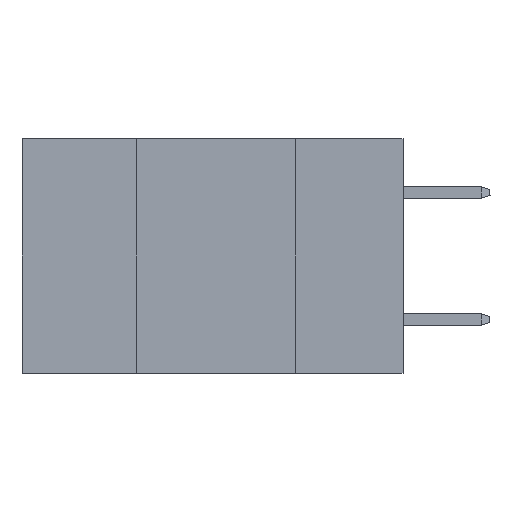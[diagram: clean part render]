
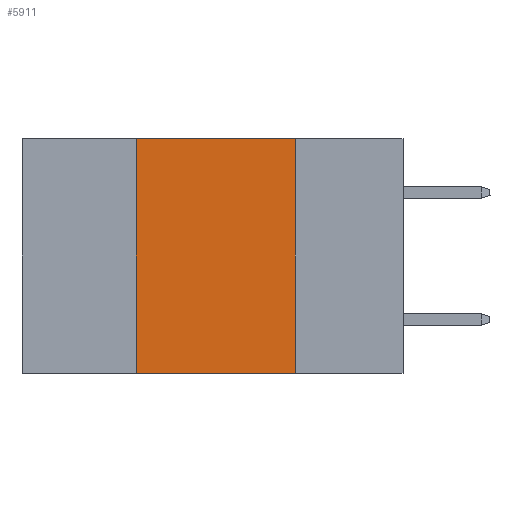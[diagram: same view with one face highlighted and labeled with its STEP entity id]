
A CAD part, left-side view. The second image highlights one B-rep face of the part: STEP entity #5911.
In plain terms, the highlighted planar face has unit normal (-1, 0, 0).
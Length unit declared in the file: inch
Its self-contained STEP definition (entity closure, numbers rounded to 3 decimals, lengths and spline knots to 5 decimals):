
#369 = CARTESIAN_POINT ( 'NONE',  ( 0., 0.42, -0.37 ) ) ;
#667 = VERTEX_POINT ( 'NONE', #26846 ) ;
#1873 = DIRECTION ( 'NONE',  ( 0., 0., 1. ) ) ;
#2934 = FACE_OUTER_BOUND ( 'NONE', #6196, .T. ) ;
#4989 = LINE ( 'NONE', #30145, #19191 ) ;
#5911 = ADVANCED_FACE ( 'NONE', ( #2934 ), #17420, .F. ) ;
#6111 = DIRECTION ( 'NONE',  ( 0., -1., 0. ) ) ;
#6196 = EDGE_LOOP ( 'NONE', ( #30304, #21961, #32910, #29564 ) ) ;
#7143 = EDGE_CURVE ( 'NONE', #31161, #16699, #19513, .T. ) ;
#8806 = DIRECTION ( 'NONE',  ( 1., 0., 0. ) ) ;
#11231 = CARTESIAN_POINT ( 'NONE',  ( 0., 0.17, -0.37 ) ) ;
#12310 = VECTOR ( 'NONE', #1873, 39.37008 ) ;
#16320 = CARTESIAN_POINT ( 'NONE',  ( 0., 0.6, -0.37 ) ) ;
#16699 = VERTEX_POINT ( 'NONE', #11231 ) ;
#17420 = PLANE ( 'NONE',  #36991 ) ;
#18185 = LINE ( 'NONE', #38845, #12310 ) ;
#19191 = VECTOR ( 'NONE', #22674, 39.37008 ) ;
#19513 = LINE ( 'NONE', #16320, #34757 ) ;
#21961 = ORIENTED_EDGE ( 'NONE', *, *, #22437, .F. ) ;
#22437 = EDGE_CURVE ( 'NONE', #667, #36093, #40378, .T. ) ;
#22674 = DIRECTION ( 'NONE',  ( 0., 0., -1. ) ) ;
#24629 = EDGE_CURVE ( 'NONE', #31161, #667, #18185, .T. ) ;
#24665 = CARTESIAN_POINT ( 'NONE',  ( 0., 0.17, 0. ) ) ;
#26737 = CARTESIAN_POINT ( 'NONE',  ( 0., 0.6, 0. ) ) ;
#26846 = CARTESIAN_POINT ( 'NONE',  ( 0., 0.42, 0. ) ) ;
#27868 = DIRECTION ( 'NONE',  ( 0., 0., -1. ) ) ;
#29564 = ORIENTED_EDGE ( 'NONE', *, *, #7143, .T. ) ;
#29944 = DIRECTION ( 'NONE',  ( 0., -1., 0. ) ) ;
#30145 = CARTESIAN_POINT ( 'NONE',  ( 0., 0.17, 0. ) ) ;
#30304 = ORIENTED_EDGE ( 'NONE', *, *, #35763, .F. ) ;
#31161 = VERTEX_POINT ( 'NONE', #369 ) ;
#32910 = ORIENTED_EDGE ( 'NONE', *, *, #24629, .F. ) ;
#34757 = VECTOR ( 'NONE', #29944, 39.37008 ) ;
#35763 = EDGE_CURVE ( 'NONE', #36093, #16699, #4989, .T. ) ;
#36093 = VERTEX_POINT ( 'NONE', #24665 ) ;
#36991 = AXIS2_PLACEMENT_3D ( 'NONE', #41921, #8806, #27868 ) ;
#38845 = CARTESIAN_POINT ( 'NONE',  ( 0., 0.42, 0. ) ) ;
#40378 = LINE ( 'NONE', #26737, #42015 ) ;
#41921 = CARTESIAN_POINT ( 'NONE',  ( 0., 0.6, 0. ) ) ;
#42015 = VECTOR ( 'NONE', #6111, 39.37008 ) ;
